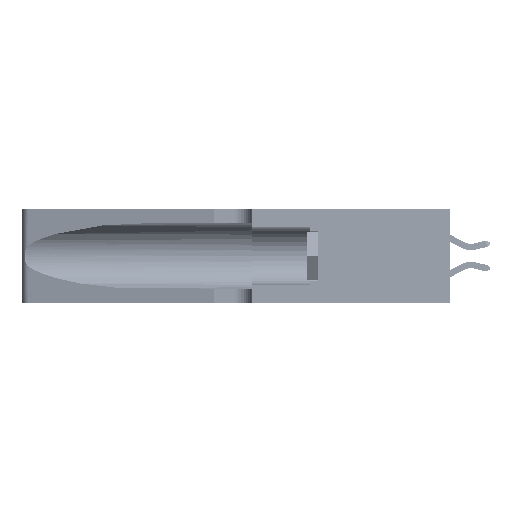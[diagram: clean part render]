
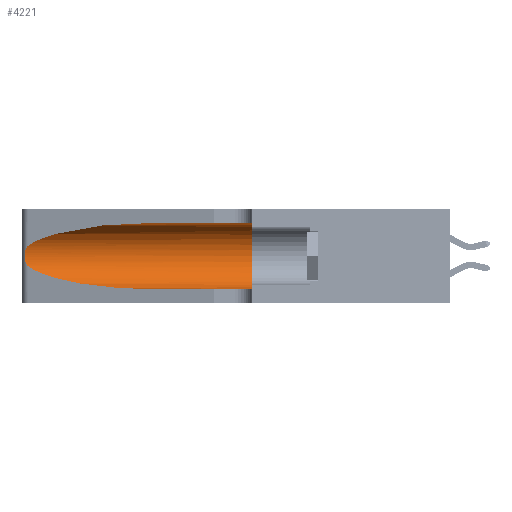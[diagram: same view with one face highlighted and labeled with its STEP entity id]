
A CAD part, left-side view. The second image highlights one B-rep face of the part: STEP entity #4221.
In plain terms, the highlighted cylindrical face has radius 3.308 mm (diameter 6.617 mm), a partial arc.
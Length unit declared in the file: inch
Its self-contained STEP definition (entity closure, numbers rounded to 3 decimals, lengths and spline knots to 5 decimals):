
#703 = ORIENTED_EDGE ( 'NONE', *, *, #5885, .T. ) ;
#1885 = CARTESIAN_POINT ( 'NONE',  ( 0.1305, 0.72297, 0.05475 ) ) ;
#2052 = CARTESIAN_POINT ( 'NONE',  ( 0.2373, 1.15595, 0.28018 ) ) ;
#2167 = EDGE_CURVE ( 'NONE', #43997, #28531, #24649, .T. ) ;
#2514 = CARTESIAN_POINT ( 'NONE',  ( 0.25487, 1.22718, 0.22369 ) ) ;
#3151 = CARTESIAN_POINT ( 'NONE',  ( 0.25487, 1.22718, 0.14631 ) ) ;
#3855 = DIRECTION ( 'NONE',  ( 0., -1., 0. ) ) ;
#4221 = ADVANCED_FACE ( 'NONE', ( #9906 ), #8600, .F. ) ;
#4465 = CARTESIAN_POINT ( 'NONE',  ( 0.1305, 0.35, 0.05475 ) ) ;
#5885 = EDGE_CURVE ( 'NONE', #17830, #27590, #18362, .T. ) ;
#6622 = CARTESIAN_POINT ( 'NONE',  ( 0.25854, 1.2359, 0.20912 ) ) ;
#6670 = CARTESIAN_POINT ( 'NONE',  ( 0.1305, 0.72297, 0.05475 ) ) ;
#8600 = CYLINDRICAL_SURFACE ( 'NONE', #37385, 0.13025 ) ;
#9452 = LINE ( 'NONE', #45881, #31019 ) ;
#9719 = ORIENTED_EDGE ( 'NONE', *, *, #2167, .F. ) ;
#9906 = FACE_OUTER_BOUND ( 'NONE', #36209, .T. ) ;
#10539 =( BOUNDED_CURVE ( )  B_SPLINE_CURVE ( 3, ( #22363, #26445, #2052, #30500 ),
 .UNSPECIFIED., .F., .F. ) 
 B_SPLINE_CURVE_WITH_KNOTS ( ( 4, 4 ),
 ( 1.5708, 2.84003 ),
 .UNSPECIFIED. ) 
 CURVE ( )  GEOMETRIC_REPRESENTATION_ITEM ( )  RATIONAL_B_SPLINE_CURVE ( ( 1., 0.87, 0.87, 1. ) ) 
 REPRESENTATION_ITEM ( '' )  );
#10733 = CARTESIAN_POINT ( 'NONE',  ( 0.26075, 1.23896, 0.19203 ) ) ;
#10947 = VERTEX_POINT ( 'NONE', #34431 ) ;
#13796 = CARTESIAN_POINT ( 'NONE',  ( 0.25487, 1.22718, 0.22369 ) ) ;
#14062 = CARTESIAN_POINT ( 'NONE',  ( 0.25487, 1.22718, 0.14631 ) ) ;
#14830 = CARTESIAN_POINT ( 'NONE',  ( 0.26017, 1.23833, 0.17102 ) ) ;
#16688 = ORIENTED_EDGE ( 'NONE', *, *, #25880, .T. ) ;
#17741 = DIRECTION ( 'NONE',  ( 0., -1., 0. ) ) ;
#17830 = VERTEX_POINT ( 'NONE', #13796 ) ;
#18362 = B_SPLINE_CURVE_WITH_KNOTS ( 'NONE', 3,
 ( #2514, #50934, #26894, #30934, #6622, #34979, #10733, #39029, #14830, #43005, #18906, #47039, #22990, #51107 ),
 .UNSPECIFIED., .F., .F.,
 ( 4, 2, 2, 2, 2, 2, 4 ),
 ( 0., 0.00027, 0.00053, 0.00107, 0.0016, 0.00187, 0.00214 ),
 .UNSPECIFIED. ) ;
#18713 = DIRECTION ( 'NONE',  ( 0., 0., -1. ) ) ;
#18906 = CARTESIAN_POINT ( 'NONE',  ( 0.25789, 1.23486, 0.15765 ) ) ;
#20532 = CARTESIAN_POINT ( 'NONE',  ( 0.1305, 0.35, 0.31525 ) ) ;
#21249 = DIRECTION ( 'NONE',  ( 0., 1., 0. ) ) ;
#22363 = CARTESIAN_POINT ( 'NONE',  ( 0.1305, 0.72297, 0.31525 ) ) ;
#22990 = CARTESIAN_POINT ( 'NONE',  ( 0.25555, 1.22993, 0.14849 ) ) ;
#23843 = VERTEX_POINT ( 'NONE', #6670 ) ;
#24649 = CIRCLE ( 'NONE', #48707, 0.13025 ) ;
#25880 = EDGE_CURVE ( 'NONE', #23843, #28531, #9452, .T. ) ;
#26221 = ORIENTED_EDGE ( 'NONE', *, *, #51747, .T. ) ;
#26274 = CARTESIAN_POINT ( 'NONE',  ( 0.18966, 0.96281, 0.05475 ) ) ;
#26445 = CARTESIAN_POINT ( 'NONE',  ( 0.18966, 0.96281, 0.31525 ) ) ;
#26894 = CARTESIAN_POINT ( 'NONE',  ( 0.25639, 1.23184, 0.21858 ) ) ;
#27590 = VERTEX_POINT ( 'NONE', #3151 ) ;
#28255 = CARTESIAN_POINT ( 'NONE',  ( 0.1305, 1.61858, 0.31525 ) ) ;
#28531 = VERTEX_POINT ( 'NONE', #4465 ) ;
#30500 = CARTESIAN_POINT ( 'NONE',  ( 0.25487, 1.22718, 0.22369 ) ) ;
#30729 = CARTESIAN_POINT ( 'NONE',  ( 0.1305, 1.61858, 0.185 ) ) ;
#30934 = CARTESIAN_POINT ( 'NONE',  ( 0.25787, 1.23484, 0.2124 ) ) ;
#31019 = VECTOR ( 'NONE', #17741, 39.37008 ) ;
#31886 = ORIENTED_EDGE ( 'NONE', *, *, #49869, .T. ) ;
#34431 = CARTESIAN_POINT ( 'NONE',  ( 0.1305, 0.72297, 0.31525 ) ) ;
#34979 = CARTESIAN_POINT ( 'NONE',  ( 0.26018, 1.23835, 0.19895 ) ) ;
#35055 = ORIENTED_EDGE ( 'NONE', *, *, #51445, .F. ) ;
#36209 = EDGE_LOOP ( 'NONE', ( #31886, #703, #26221, #16688, #9719, #35055 ) ) ;
#37385 = AXIS2_PLACEMENT_3D ( 'NONE', #30729, #42799, #18713 ) ;
#39029 = CARTESIAN_POINT ( 'NONE',  ( 0.26075, 1.23896, 0.178 ) ) ;
#42799 = DIRECTION ( 'NONE',  ( 0., -1., 0. ) ) ;
#43005 = CARTESIAN_POINT ( 'NONE',  ( 0.25856, 1.23593, 0.16098 ) ) ;
#43997 = VERTEX_POINT ( 'NONE', #20532 ) ;
#44130 =( BOUNDED_CURVE ( )  B_SPLINE_CURVE ( 3, ( #14062, #46258, #26274, #1885 ),
 .UNSPECIFIED., .F., .F. ) 
 B_SPLINE_CURVE_WITH_KNOTS ( ( 4, 4 ),
 ( 3.44316, 4.71239 ),
 .UNSPECIFIED. ) 
 CURVE ( )  GEOMETRIC_REPRESENTATION_ITEM ( )  RATIONAL_B_SPLINE_CURVE ( ( 1., 0.87, 0.87, 1. ) ) 
 REPRESENTATION_ITEM ( '' )  );
#44336 = VECTOR ( 'NONE', #3855, 39.37008 ) ;
#45329 = CARTESIAN_POINT ( 'NONE',  ( 0.1305, 0.35, 0.185 ) ) ;
#45605 = LINE ( 'NONE', #28255, #44336 ) ;
#45881 = CARTESIAN_POINT ( 'NONE',  ( 0.1305, 1.61858, 0.05475 ) ) ;
#46258 = CARTESIAN_POINT ( 'NONE',  ( 0.2373, 1.15595, 0.08982 ) ) ;
#47039 = CARTESIAN_POINT ( 'NONE',  ( 0.25639, 1.23186, 0.15144 ) ) ;
#48707 = AXIS2_PLACEMENT_3D ( 'NONE', #45329, #21249, #49378 ) ;
#49378 = DIRECTION ( 'NONE',  ( 0., 0., 1. ) ) ;
#49869 = EDGE_CURVE ( 'NONE', #10947, #17830, #10539, .T. ) ;
#50934 = CARTESIAN_POINT ( 'NONE',  ( 0.25555, 1.22994, 0.2215 ) ) ;
#51107 = CARTESIAN_POINT ( 'NONE',  ( 0.25487, 1.22718, 0.14631 ) ) ;
#51445 = EDGE_CURVE ( 'NONE', #10947, #43997, #45605, .T. ) ;
#51747 = EDGE_CURVE ( 'NONE', #27590, #23843, #44130, .T. ) ;
